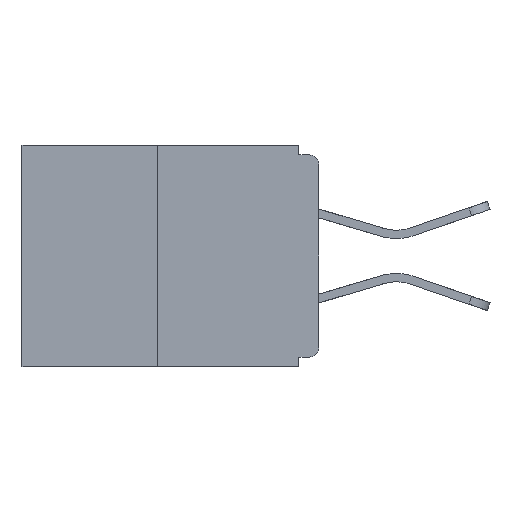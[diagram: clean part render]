
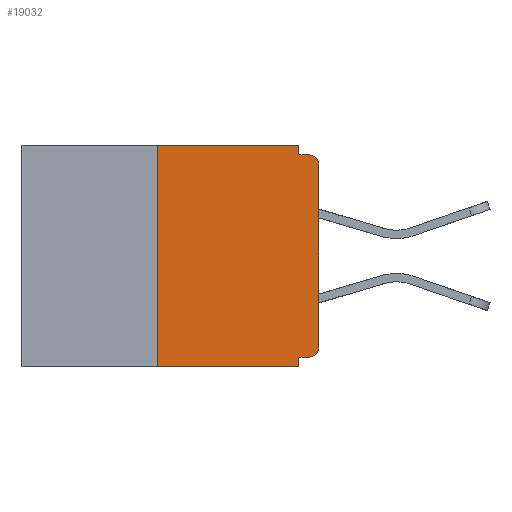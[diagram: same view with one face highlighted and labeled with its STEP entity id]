
A CAD part, left-side view. The second image highlights one B-rep face of the part: STEP entity #19032.
In plain terms, the highlighted planar face has unit normal (-1, 0, 0).
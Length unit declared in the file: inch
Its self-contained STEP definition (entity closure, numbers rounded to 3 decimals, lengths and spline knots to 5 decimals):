
#106 = EDGE_CURVE ( 'NONE', #9106, #11766, #8515, .T. ) ;
#804 = CARTESIAN_POINT ( 'NONE',  ( 0., 0.031, 0. ) ) ;
#889 = VERTEX_POINT ( 'NONE', #30634 ) ;
#921 = ORIENTED_EDGE ( 'NONE', *, *, #19277, .T. ) ;
#1203 = VECTOR ( 'NONE', #14357, 39.37008 ) ;
#1300 = DIRECTION ( 'NONE',  ( 0., 1., 0. ) ) ;
#1326 = VECTOR ( 'NONE', #1300, 39.37008 ) ;
#1500 = AXIS2_PLACEMENT_3D ( 'NONE', #8199, #3288, #24950 ) ;
#1585 = DIRECTION ( 'NONE',  ( 0., -1., 0. ) ) ;
#1761 = CARTESIAN_POINT ( 'NONE',  ( 0., 0.015, -0.328 ) ) ;
#1974 = CARTESIAN_POINT ( 'NONE',  ( 0., 0.031, -0.015 ) ) ;
#2375 = CARTESIAN_POINT ( 'NONE',  ( 0., 0.015, -0.313 ) ) ;
#3288 = DIRECTION ( 'NONE',  ( 1., 0., 0. ) ) ;
#3338 = VECTOR ( 'NONE', #1585, 39.37008 ) ;
#5219 = EDGE_CURVE ( 'NONE', #21362, #23636, #23969, .T. ) ;
#5247 = EDGE_CURVE ( 'NONE', #889, #21558, #19820, .T. ) ;
#5248 = VECTOR ( 'NONE', #16443, 39.37008 ) ;
#5951 = ORIENTED_EDGE ( 'NONE', *, *, #5219, .F. ) ;
#6104 = VERTEX_POINT ( 'NONE', #17945 ) ;
#6307 = ORIENTED_EDGE ( 'NONE', *, *, #19770, .T. ) ;
#7573 = LINE ( 'NONE', #11297, #29629 ) ;
#7968 = ORIENTED_EDGE ( 'NONE', *, *, #19825, .F. ) ;
#8025 = ORIENTED_EDGE ( 'NONE', *, *, #30478, .F. ) ;
#8199 = CARTESIAN_POINT ( 'NONE',  ( 0., 0.46, 0. ) ) ;
#8515 = LINE ( 'NONE', #10537, #29840 ) ;
#8590 = VECTOR ( 'NONE', #16143, 39.37008 ) ;
#8749 = AXIS2_PLACEMENT_3D ( 'NONE', #25060, #27047, #10716 ) ;
#8881 = VECTOR ( 'NONE', #19967, 39.37008 ) ;
#9106 = VERTEX_POINT ( 'NONE', #9127 ) ;
#9127 = CARTESIAN_POINT ( 'NONE',  ( 0., 0.25, -0.343 ) ) ;
#9608 = DIRECTION ( 'NONE',  ( 0., 0., -1. ) ) ;
#10232 = CARTESIAN_POINT ( 'NONE',  ( 0., 0.031, -0.343 ) ) ;
#10537 = CARTESIAN_POINT ( 'NONE',  ( 0., 0.46, -0.343 ) ) ;
#10716 = DIRECTION ( 'NONE',  ( 0., 0., -1. ) ) ;
#11297 = CARTESIAN_POINT ( 'NONE',  ( 0., 0.25, 0. ) ) ;
#11719 = DIRECTION ( 'NONE',  ( 0., 0., 1. ) ) ;
#11766 = VERTEX_POINT ( 'NONE', #24602 ) ;
#12566 = LINE ( 'NONE', #15755, #1326 ) ;
#13549 = EDGE_CURVE ( 'NONE', #9106, #6104, #7573, .T. ) ;
#13630 = CARTESIAN_POINT ( 'NONE',  ( 0., 0., 0. ) ) ;
#13687 = ORIENTED_EDGE ( 'NONE', *, *, #106, .T. ) ;
#13886 = ORIENTED_EDGE ( 'NONE', *, *, #21668, .F. ) ;
#14096 = CIRCLE ( 'NONE', #8749, 0.015 ) ;
#14357 = DIRECTION ( 'NONE',  ( 0., 0., -1. ) ) ;
#14374 = LINE ( 'NONE', #14555, #1203 ) ;
#14555 = CARTESIAN_POINT ( 'NONE',  ( 0., 0.031, 0. ) ) ;
#14602 = AXIS2_PLACEMENT_3D ( 'NONE', #2375, #23961, #9608 ) ;
#15755 = CARTESIAN_POINT ( 'NONE',  ( 0., 0., -0.328 ) ) ;
#16017 = CARTESIAN_POINT ( 'NONE',  ( 0., 0.46, 0. ) ) ;
#16143 = DIRECTION ( 'NONE',  ( 0., 0., 1. ) ) ;
#16443 = DIRECTION ( 'NONE',  ( 0., -1., 0. ) ) ;
#16991 = VERTEX_POINT ( 'NONE', #1761 ) ;
#17931 = CARTESIAN_POINT ( 'NONE',  ( 0., 0., -0.03 ) ) ;
#17945 = CARTESIAN_POINT ( 'NONE',  ( 0., 0.25, 0. ) ) ;
#19032 = ADVANCED_FACE ( 'NONE', ( #29443 ), #22578, .F. ) ;
#19277 = EDGE_CURVE ( 'NONE', #16991, #889, #21613, .T. ) ;
#19446 = ORIENTED_EDGE ( 'NONE', *, *, #5247, .T. ) ;
#19770 = EDGE_CURVE ( 'NONE', #21558, #23636, #14096, .T. ) ;
#19820 = LINE ( 'NONE', #13630, #8590 ) ;
#19825 = EDGE_CURVE ( 'NONE', #16991, #27016, #12566, .T. ) ;
#19967 = DIRECTION ( 'NONE',  ( 0., 0., -1. ) ) ;
#21046 = CARTESIAN_POINT ( 'NONE',  ( 0., 0.031, -0.328 ) ) ;
#21362 = VERTEX_POINT ( 'NONE', #1974 ) ;
#21558 = VERTEX_POINT ( 'NONE', #17931 ) ;
#21613 = CIRCLE ( 'NONE', #14602, 0.015 ) ;
#21668 = EDGE_CURVE ( 'NONE', #21985, #21362, #14374, .T. ) ;
#21985 = VERTEX_POINT ( 'NONE', #804 ) ;
#22367 = ORIENTED_EDGE ( 'NONE', *, *, #23823, .F. ) ;
#22578 = PLANE ( 'NONE',  #1500 ) ;
#22722 = ORIENTED_EDGE ( 'NONE', *, *, #13549, .F. ) ;
#23636 = VERTEX_POINT ( 'NONE', #25425 ) ;
#23823 = EDGE_CURVE ( 'NONE', #6104, #21985, #28789, .T. ) ;
#23961 = DIRECTION ( 'NONE',  ( -1., 0., 0. ) ) ;
#23969 = LINE ( 'NONE', #27919, #3338 ) ;
#24602 = CARTESIAN_POINT ( 'NONE',  ( 0., 0.031, -0.343 ) ) ;
#24950 = DIRECTION ( 'NONE',  ( 0., 0., -1. ) ) ;
#25060 = CARTESIAN_POINT ( 'NONE',  ( 0., 0.015, -0.03 ) ) ;
#25425 = CARTESIAN_POINT ( 'NONE',  ( 0., 0.015, -0.015 ) ) ;
#25736 = LINE ( 'NONE', #10232, #8881 ) ;
#26481 = EDGE_LOOP ( 'NONE', ( #22367, #22722, #13687, #8025, #7968, #921, #19446, #6307, #5951, #13886 ) ) ;
#26959 = DIRECTION ( 'NONE',  ( 0., -1., 0. ) ) ;
#27016 = VERTEX_POINT ( 'NONE', #21046 ) ;
#27047 = DIRECTION ( 'NONE',  ( -1., 0., 0. ) ) ;
#27919 = CARTESIAN_POINT ( 'NONE',  ( 0., 0., -0.015 ) ) ;
#28789 = LINE ( 'NONE', #16017, #5248 ) ;
#29443 = FACE_OUTER_BOUND ( 'NONE', #26481, .T. ) ;
#29629 = VECTOR ( 'NONE', #11719, 39.37008 ) ;
#29840 = VECTOR ( 'NONE', #26959, 39.37008 ) ;
#30478 = EDGE_CURVE ( 'NONE', #27016, #11766, #25736, .T. ) ;
#30634 = CARTESIAN_POINT ( 'NONE',  ( 0., 0., -0.313 ) ) ;
